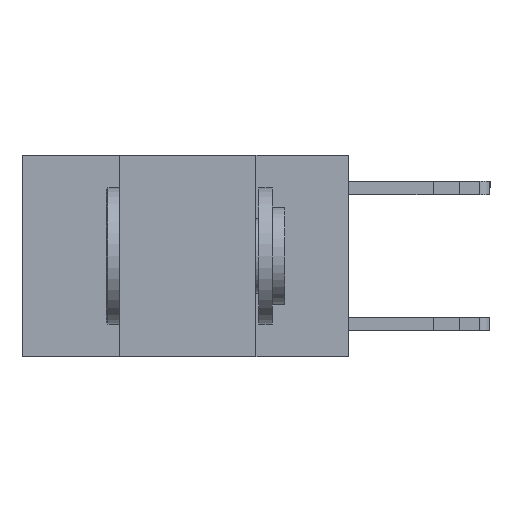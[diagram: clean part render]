
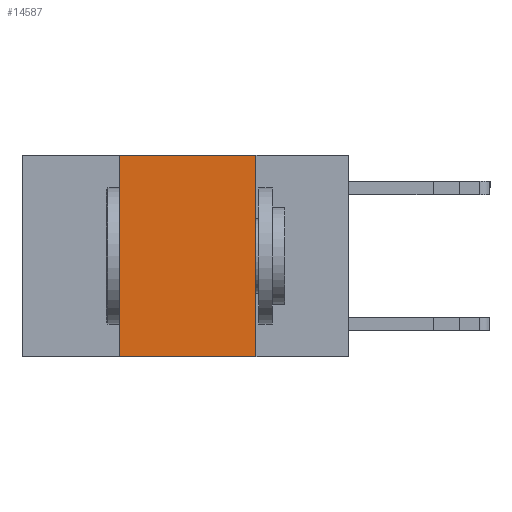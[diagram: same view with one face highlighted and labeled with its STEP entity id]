
A CAD part, left-side view. The second image highlights one B-rep face of the part: STEP entity #14587.
In plain terms, the highlighted planar face has unit normal (-1, 0, 0).
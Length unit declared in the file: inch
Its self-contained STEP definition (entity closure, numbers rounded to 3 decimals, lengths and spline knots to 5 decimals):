
#174 = FACE_OUTER_BOUND ( 'NONE', #10366, .T. ) ;
#792 = VECTOR ( 'NONE', #3529, 39.37008 ) ;
#1204 = EDGE_CURVE ( 'NONE', #11378, #1731, #17134, .T. ) ;
#1277 = VERTEX_POINT ( 'NONE', #15291 ) ;
#1731 = VERTEX_POINT ( 'NONE', #14197 ) ;
#1820 = CARTESIAN_POINT ( 'NONE',  ( 0., 0.42, 0. ) ) ;
#3447 = AXIS2_PLACEMENT_3D ( 'NONE', #9392, #15765, #6290 ) ;
#3529 = DIRECTION ( 'NONE',  ( 0., -1., 0. ) ) ;
#5487 = EDGE_CURVE ( 'NONE', #1277, #11378, #13605, .T. ) ;
#6062 = DIRECTION ( 'NONE',  ( 0., 0., 1. ) ) ;
#6290 = DIRECTION ( 'NONE',  ( 0., 0., -1. ) ) ;
#6350 = DIRECTION ( 'NONE',  ( 0., -1., 0. ) ) ;
#6384 = PLANE ( 'NONE',  #3447 ) ;
#7455 = ORIENTED_EDGE ( 'NONE', *, *, #5487, .F. ) ;
#7519 = CARTESIAN_POINT ( 'NONE',  ( 0., 0.17, 0. ) ) ;
#9392 = CARTESIAN_POINT ( 'NONE',  ( 0., 0.6, 0. ) ) ;
#9695 = VECTOR ( 'NONE', #6062, 39.37008 ) ;
#10366 = EDGE_LOOP ( 'NONE', ( #11351, #7455, #16876, #15797 ) ) ;
#11351 = ORIENTED_EDGE ( 'NONE', *, *, #1204, .F. ) ;
#11378 = VERTEX_POINT ( 'NONE', #7519 ) ;
#11992 = DIRECTION ( 'NONE',  ( 0., 0., -1. ) ) ;
#12624 = CARTESIAN_POINT ( 'NONE',  ( 0., 0.42, -0.37 ) ) ;
#13605 = LINE ( 'NONE', #19874, #17899 ) ;
#13737 = EDGE_CURVE ( 'NONE', #19477, #1731, #17566, .T. ) ;
#14197 = CARTESIAN_POINT ( 'NONE',  ( 0., 0.17, -0.37 ) ) ;
#14411 = LINE ( 'NONE', #1820, #9695 ) ;
#14476 = VECTOR ( 'NONE', #11992, 39.37008 ) ;
#14587 = ADVANCED_FACE ( 'NONE', ( #174 ), #6384, .F. ) ;
#15029 = EDGE_CURVE ( 'NONE', #19477, #1277, #14411, .T. ) ;
#15291 = CARTESIAN_POINT ( 'NONE',  ( 0., 0.42, 0. ) ) ;
#15765 = DIRECTION ( 'NONE',  ( 1., 0., 0. ) ) ;
#15797 = ORIENTED_EDGE ( 'NONE', *, *, #13737, .T. ) ;
#16717 = CARTESIAN_POINT ( 'NONE',  ( 0., 0.17, 0. ) ) ;
#16876 = ORIENTED_EDGE ( 'NONE', *, *, #15029, .F. ) ;
#17134 = LINE ( 'NONE', #16717, #14476 ) ;
#17566 = LINE ( 'NONE', #17666, #792 ) ;
#17666 = CARTESIAN_POINT ( 'NONE',  ( 0., 0.6, -0.37 ) ) ;
#17899 = VECTOR ( 'NONE', #6350, 39.37008 ) ;
#19477 = VERTEX_POINT ( 'NONE', #12624 ) ;
#19874 = CARTESIAN_POINT ( 'NONE',  ( 0., 0.6, 0. ) ) ;
